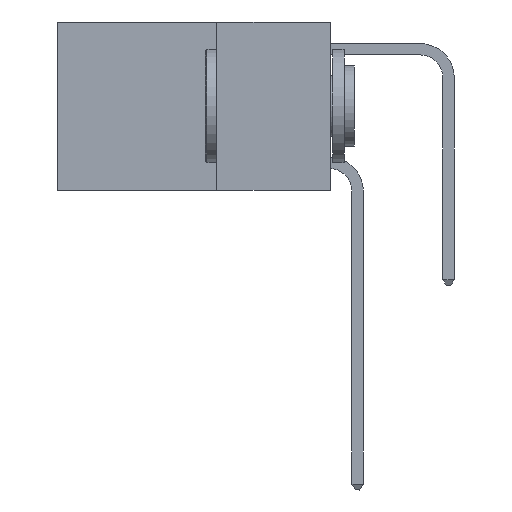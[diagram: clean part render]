
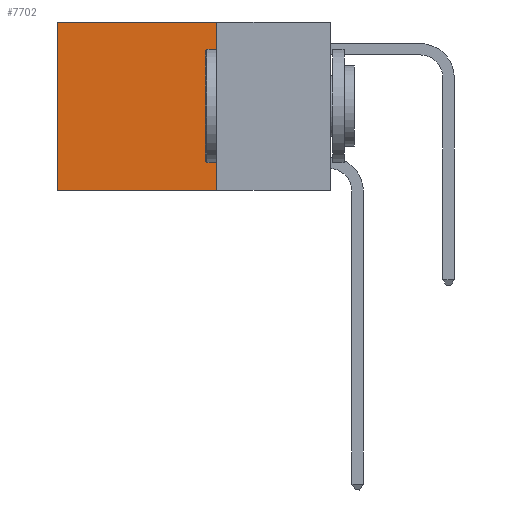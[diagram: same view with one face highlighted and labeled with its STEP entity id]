
A CAD part, left-side view. The second image highlights one B-rep face of the part: STEP entity #7702.
In plain terms, the highlighted planar face has unit normal (-1, 0, 0).
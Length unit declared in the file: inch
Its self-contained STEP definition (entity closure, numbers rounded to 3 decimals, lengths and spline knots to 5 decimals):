
#214 = EDGE_CURVE ( 'NONE', #16150, #5108, #12125, .T. ) ;
#1082 = CARTESIAN_POINT ( 'NONE',  ( 0.2625, 0.25, -0.37 ) ) ;
#1830 = DIRECTION ( 'NONE',  ( 0., 1., 0. ) ) ;
#2875 = CARTESIAN_POINT ( 'NONE',  ( 0.2625, 0.25, 0. ) ) ;
#4753 = VECTOR ( 'NONE', #15981, 39.37008 ) ;
#5108 = VERTEX_POINT ( 'NONE', #13111 ) ;
#5606 = LINE ( 'NONE', #13184, #16287 ) ;
#5991 = DIRECTION ( 'NONE',  ( 0., 1., 0. ) ) ;
#7160 = EDGE_LOOP ( 'NONE', ( #17094, #19331, #7726, #21647 ) ) ;
#7702 = ADVANCED_FACE ( 'NONE', ( #11722 ), #19879, .F. ) ;
#7726 = ORIENTED_EDGE ( 'NONE', *, *, #8017, .F. ) ;
#8017 = EDGE_CURVE ( 'NONE', #20842, #19854, #19424, .T. ) ;
#10526 = DIRECTION ( 'NONE',  ( 0., 0., -1. ) ) ;
#11468 = DIRECTION ( 'NONE',  ( 1., 0., 0. ) ) ;
#11483 = AXIS2_PLACEMENT_3D ( 'NONE', #2875, #11468, #18237 ) ;
#11722 = FACE_OUTER_BOUND ( 'NONE', #7160, .T. ) ;
#11893 = EDGE_CURVE ( 'NONE', #19854, #5108, #17400, .T. ) ;
#12125 = LINE ( 'NONE', #15203, #17705 ) ;
#13031 = EDGE_CURVE ( 'NONE', #20842, #16150, #5606, .T. ) ;
#13111 = CARTESIAN_POINT ( 'NONE',  ( 0.2625, 0.6, -0.37 ) ) ;
#13184 = CARTESIAN_POINT ( 'NONE',  ( 0.2625, 0.25, 0. ) ) ;
#13960 = VECTOR ( 'NONE', #5991, 39.37008 ) ;
#14169 = CARTESIAN_POINT ( 'NONE',  ( 0.2625, 0.25, -0.37 ) ) ;
#15140 = CARTESIAN_POINT ( 'NONE',  ( 0.2625, 0.6, 0. ) ) ;
#15203 = CARTESIAN_POINT ( 'NONE',  ( 0.2625, 0.6, 0. ) ) ;
#15981 = DIRECTION ( 'NONE',  ( 0., 0., -1. ) ) ;
#16150 = VERTEX_POINT ( 'NONE', #15140 ) ;
#16287 = VECTOR ( 'NONE', #1830, 39.37008 ) ;
#17094 = ORIENTED_EDGE ( 'NONE', *, *, #214, .T. ) ;
#17400 = LINE ( 'NONE', #1082, #13960 ) ;
#17705 = VECTOR ( 'NONE', #10526, 39.37008 ) ;
#18237 = DIRECTION ( 'NONE',  ( 0., 0., -1. ) ) ;
#19146 = CARTESIAN_POINT ( 'NONE',  ( 0.2625, 0.25, 0. ) ) ;
#19194 = CARTESIAN_POINT ( 'NONE',  ( 0.2625, 0.25, 0. ) ) ;
#19331 = ORIENTED_EDGE ( 'NONE', *, *, #11893, .F. ) ;
#19424 = LINE ( 'NONE', #19194, #4753 ) ;
#19854 = VERTEX_POINT ( 'NONE', #14169 ) ;
#19879 = PLANE ( 'NONE',  #11483 ) ;
#20842 = VERTEX_POINT ( 'NONE', #19146 ) ;
#21647 = ORIENTED_EDGE ( 'NONE', *, *, #13031, .T. ) ;
